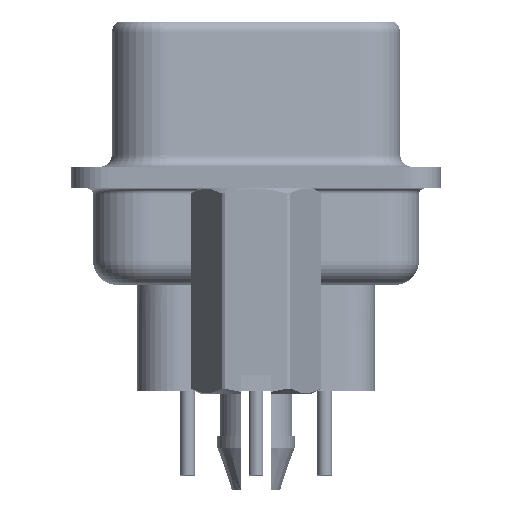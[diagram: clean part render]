
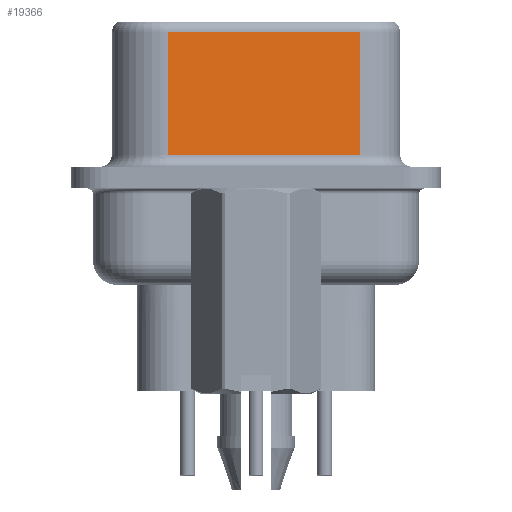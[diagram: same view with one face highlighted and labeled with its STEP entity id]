
A CAD part, left-side view. The second image highlights one B-rep face of the part: STEP entity #19366.
In plain terms, the highlighted planar face has unit normal (-0.985, -0.174, 0).
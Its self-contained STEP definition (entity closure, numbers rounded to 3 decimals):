
#29 = LINE ( 'NONE', #44514, #42178 ) ;
#94 = CARTESIAN_POINT ( 'NONE',  ( 3.73, 3.628, 6.52 ) ) ;
#291 = EDGE_LOOP ( 'NONE', ( #17491, #8618, #51699, #8763 ) ) ;
#2558 = EDGE_CURVE ( 'NONE', #17795, #44959, #56633, .T. ) ;
#4194 = EDGE_CURVE ( 'NONE', #44959, #39368, #34595, .T. ) ;
#5783 = VERTEX_POINT ( 'NONE', #56568 ) ;
#5995 = EDGE_CURVE ( 'NONE', #5783, #39368, #29, .T. ) ;
#8551 = CARTESIAN_POINT ( 'NONE',  ( 5.132, -4.322, 0.95 ) ) ;
#8618 = ORIENTED_EDGE ( 'NONE', *, *, #55041, .T. ) ;
#8763 = ORIENTED_EDGE ( 'NONE', *, *, #4194, .T. ) ;
#9473 = CARTESIAN_POINT ( 'NONE',  ( 5.132, -4.322, 6.02 ) ) ;
#17491 = ORIENTED_EDGE ( 'NONE', *, *, #5995, .F. ) ;
#17795 = VERTEX_POINT ( 'NONE', #42792 ) ;
#17889 = VECTOR ( 'NONE', #30250, 1000. ) ;
#19366 = ADVANCED_FACE ( 'NONE', ( #21594 ), #43119, .F. ) ;
#21594 = FACE_OUTER_BOUND ( 'NONE', #291, .T. ) ;
#25156 = CARTESIAN_POINT ( 'NONE',  ( 5.132, -4.322, 0.95 ) ) ;
#25365 = DIRECTION ( 'NONE',  ( 0.985, 0.174, 0. ) ) ;
#30220 = CARTESIAN_POINT ( 'NONE',  ( 5.132, -4.322, 6.52 ) ) ;
#30250 = DIRECTION ( 'NONE',  ( 0., 0., -1. ) ) ;
#30578 = CARTESIAN_POINT ( 'NONE',  ( 3.73, 3.628, 0.95 ) ) ;
#34595 = LINE ( 'NONE', #25156, #43003 ) ;
#39368 = VERTEX_POINT ( 'NONE', #8551 ) ;
#39752 = VECTOR ( 'NONE', #40725, 1000. ) ;
#40725 = DIRECTION ( 'NONE',  ( -0.174, 0.985, 0. ) ) ;
#42178 = VECTOR ( 'NONE', #53405, 1000. ) ;
#42792 = CARTESIAN_POINT ( 'NONE',  ( 3.73, 3.628, 6.02 ) ) ;
#43003 = VECTOR ( 'NONE', #48085, 1000. ) ;
#43119 = PLANE ( 'NONE',  #45680 ) ;
#44514 = CARTESIAN_POINT ( 'NONE',  ( 5.132, -4.322, 6.52 ) ) ;
#44959 = VERTEX_POINT ( 'NONE', #30578 ) ;
#45680 = AXIS2_PLACEMENT_3D ( 'NONE', #30220, #25365, #47722 ) ;
#47722 = DIRECTION ( 'NONE',  ( -0.174, 0.985, 0. ) ) ;
#48085 = DIRECTION ( 'NONE',  ( 0.174, -0.985, 0. ) ) ;
#48790 = LINE ( 'NONE', #9473, #39752 ) ;
#51699 = ORIENTED_EDGE ( 'NONE', *, *, #2558, .T. ) ;
#53405 = DIRECTION ( 'NONE',  ( 0., 0., -1. ) ) ;
#55041 = EDGE_CURVE ( 'NONE', #5783, #17795, #48790, .T. ) ;
#56568 = CARTESIAN_POINT ( 'NONE',  ( 5.132, -4.322, 6.02 ) ) ;
#56633 = LINE ( 'NONE', #94, #17889 ) ;
